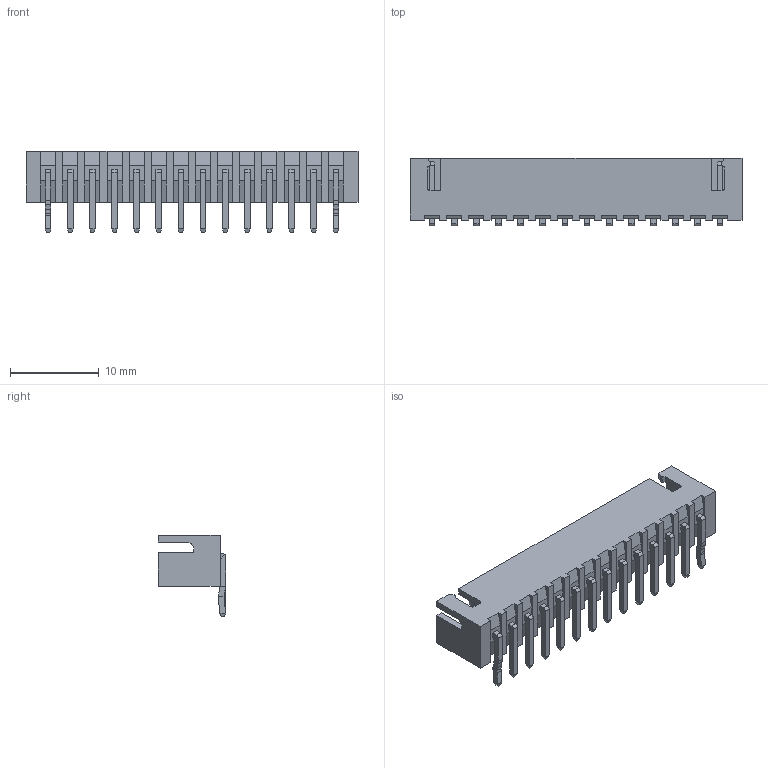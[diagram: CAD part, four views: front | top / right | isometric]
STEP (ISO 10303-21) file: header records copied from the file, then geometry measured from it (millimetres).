
FILE_DESCRIPTION (( 'STEP AP203' ), '1' );
FILE_NAME ('14K-514-421-AA1.STEP', '2024-02-23T18:07:30', ( '' ), ( '' ), 'SwSTEP 2.0', 'SolidWorks 2023', '' );
FILE_SCHEMA (( 'CONFIG_CONTROL_DESIGN' ));
Length unit declared in the file: millimetre
Products named in the file (4): 14K Series Pin_16; 14K Series Pin Header Insulator_514; 14K Series Pin_21; 14K-514-421-AA1
Assembly tree (15 placements, depth 2):
  14K-514-421-AA1
    14K Series Pin Header Insulator_514
    14K Series Pin_21  x2
    14K Series Pin_16  x12
Bounding box: 37.5 x 7.64 x 9.17 mm (x, y, z)
Volume: 712.9 mm3; surface area: 2012.5 mm2
Topology: 15 solids, 15 shells, 516 faces, 1346 edges, 860 vertices
Faces by surface type: plane 467, cylinder 49
Entity records: 8484 total; most frequent: CARTESIAN_POINT 1384, ORIENTED_EDGE 1360, DIRECTION 1246, EDGE_CURVE 680, LINE 626, VECTOR 626, VERTEX_POINT 448, AXIS2_PLACEMENT_3D 310
